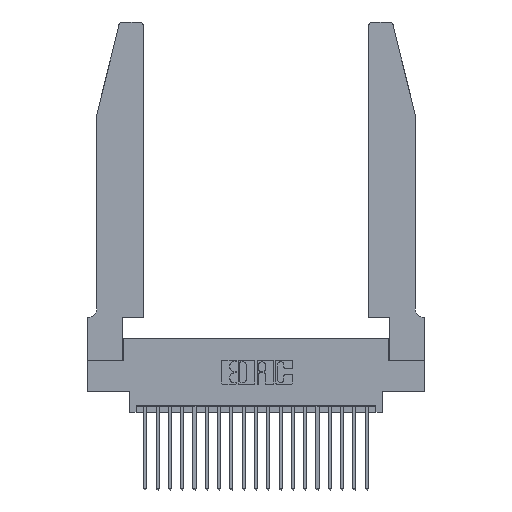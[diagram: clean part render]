
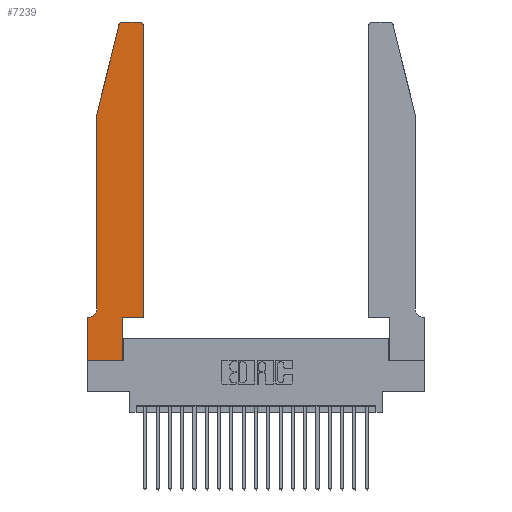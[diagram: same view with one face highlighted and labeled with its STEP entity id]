
A CAD part, top view. The second image highlights one B-rep face of the part: STEP entity #7239.
In plain terms, the highlighted planar face has unit normal (0, 0, 1).
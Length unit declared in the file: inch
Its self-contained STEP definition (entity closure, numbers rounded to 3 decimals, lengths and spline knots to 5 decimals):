
#53 = EDGE_CURVE ( 'NONE', #16785, #1456, #14814, .T. ) ;
#444 = EDGE_CURVE ( 'NONE', #21733, #634, #7860, .T. ) ;
#532 = VECTOR ( 'NONE', #2374, 39.37008 ) ;
#634 = VERTEX_POINT ( 'NONE', #20875 ) ;
#660 = ORIENTED_EDGE ( 'NONE', *, *, #5342, .T. ) ;
#842 = ORIENTED_EDGE ( 'NONE', *, *, #3606, .T. ) ;
#1038 = DIRECTION ( 'NONE',  ( 1., 0., 0. ) ) ;
#1308 = LINE ( 'NONE', #10393, #10148 ) ;
#1456 = VERTEX_POINT ( 'NONE', #11533 ) ;
#1581 = VERTEX_POINT ( 'NONE', #22406 ) ;
#1708 = AXIS2_PLACEMENT_3D ( 'NONE', #15107, #22049, #1038 ) ;
#1894 = LINE ( 'NONE', #17674, #11570 ) ;
#2374 = DIRECTION ( 'NONE',  ( 0., -1., 0. ) ) ;
#2463 = ORIENTED_EDGE ( 'NONE', *, *, #5434, .T. ) ;
#2608 = VECTOR ( 'NONE', #3742, 39.37008 ) ;
#2721 = DIRECTION ( 'NONE',  ( 1., 0., 0. ) ) ;
#3547 = EDGE_CURVE ( 'NONE', #13281, #9578, #3882, .T. ) ;
#3550 = ORIENTED_EDGE ( 'NONE', *, *, #53, .T. ) ;
#3606 = EDGE_CURVE ( 'NONE', #634, #3725, #22374, .T. ) ;
#3725 = VERTEX_POINT ( 'NONE', #6232 ) ;
#3742 = DIRECTION ( 'NONE',  ( -1., 0., 0. ) ) ;
#3859 = VERTEX_POINT ( 'NONE', #18999 ) ;
#3866 = VECTOR ( 'NONE', #10265, 39.37008 ) ;
#3882 = CIRCLE ( 'NONE', #7506, 0.03 ) ;
#4142 = ORIENTED_EDGE ( 'NONE', *, *, #4874, .T. ) ;
#4759 = CARTESIAN_POINT ( 'NONE',  ( 0.4505, 2.72, 0.37 ) ) ;
#4874 = EDGE_CURVE ( 'NONE', #1456, #13281, #1894, .T. ) ;
#5218 = DIRECTION ( 'NONE',  ( -0.239, -0.971, 0. ) ) ;
#5234 = LINE ( 'NONE', #17167, #3866 ) ;
#5342 = EDGE_CURVE ( 'NONE', #13458, #5376, #5234, .T. ) ;
#5376 = VERTEX_POINT ( 'NONE', #13996 ) ;
#5434 = EDGE_CURVE ( 'NONE', #3725, #13458, #5494, .T. ) ;
#5494 = LINE ( 'NONE', #6932, #11308 ) ;
#5713 = CARTESIAN_POINT ( 'NONE',  ( 0.0755, 0.42, 0.37 ) ) ;
#6232 = CARTESIAN_POINT ( 'NONE',  ( 0., 0., 0.37 ) ) ;
#6354 = EDGE_CURVE ( 'NONE', #9578, #3859, #1308, .T. ) ;
#6702 = EDGE_LOOP ( 'NONE', ( #4142, #7648, #18401, #22657, #6912, #9147, #842, #2463, #660, #22860, #15437, #3550 ) ) ;
#6714 = CARTESIAN_POINT ( 'NONE',  ( 0.2865, 0., 0.37 ) ) ;
#6912 = ORIENTED_EDGE ( 'NONE', *, *, #7678, .T. ) ;
#6932 = CARTESIAN_POINT ( 'NONE',  ( 0., 0., 0.37 ) ) ;
#7239 = ADVANCED_FACE ( 'NONE', ( #18969 ), #7376, .T. ) ;
#7376 = PLANE ( 'NONE',  #9772 ) ;
#7421 = CARTESIAN_POINT ( 'NONE',  ( 0.0755, 0.35, 0.37 ) ) ;
#7506 = AXIS2_PLACEMENT_3D ( 'NONE', #21258, #10679, #17708 ) ;
#7648 = ORIENTED_EDGE ( 'NONE', *, *, #3547, .T. ) ;
#7678 = EDGE_CURVE ( 'NONE', #16403, #21733, #15916, .T. ) ;
#7860 = LINE ( 'NONE', #7421, #2608 ) ;
#7906 = EDGE_CURVE ( 'NONE', #5376, #1581, #19776, .T. ) ;
#8090 = DIRECTION ( 'NONE',  ( 0., -1., 0. ) ) ;
#8780 = AXIS2_PLACEMENT_3D ( 'NONE', #10728, #22035, #14647 ) ;
#8849 = LINE ( 'NONE', #22596, #22672 ) ;
#9045 = DIRECTION ( 'NONE',  ( 1., 0., 0. ) ) ;
#9114 = CARTESIAN_POINT ( 'NONE',  ( 0., 0., 0.37 ) ) ;
#9147 = ORIENTED_EDGE ( 'NONE', *, *, #444, .T. ) ;
#9332 = CARTESIAN_POINT ( 'NONE',  ( 0.0055, 0.35, 0.37 ) ) ;
#9578 = VERTEX_POINT ( 'NONE', #19442 ) ;
#9772 = AXIS2_PLACEMENT_3D ( 'NONE', #19693, #18348, #13043 ) ;
#10148 = VECTOR ( 'NONE', #5218, 39.37008 ) ;
#10265 = DIRECTION ( 'NONE',  ( 0., 1., 0. ) ) ;
#10393 = CARTESIAN_POINT ( 'NONE',  ( 0.0755, 2., 0.37 ) ) ;
#10626 = CARTESIAN_POINT ( 'NONE',  ( 0.284, 2.75, 0.37 ) ) ;
#10679 = DIRECTION ( 'NONE',  ( 0., 0., 1. ) ) ;
#10728 = CARTESIAN_POINT ( 'NONE',  ( 0.0055, 0.42, 0.37 ) ) ;
#11308 = VECTOR ( 'NONE', #9045, 39.37008 ) ;
#11533 = CARTESIAN_POINT ( 'NONE',  ( 0.4205, 2.75, 0.37 ) ) ;
#11570 = VECTOR ( 'NONE', #21225, 39.37008 ) ;
#12288 = EDGE_CURVE ( 'NONE', #3859, #16403, #16810, .T. ) ;
#12691 = VECTOR ( 'NONE', #8090, 39.37008 ) ;
#13043 = DIRECTION ( 'NONE',  ( 1., 0., 0. ) ) ;
#13281 = VERTEX_POINT ( 'NONE', #10626 ) ;
#13458 = VERTEX_POINT ( 'NONE', #6714 ) ;
#13996 = CARTESIAN_POINT ( 'NONE',  ( 0.2865, 0.35, 0.37 ) ) ;
#14112 = DIRECTION ( 'NONE',  ( 0., 1., 0. ) ) ;
#14304 = CARTESIAN_POINT ( 'NONE',  ( 0.4505, 0.35, 0.37 ) ) ;
#14524 = VECTOR ( 'NONE', #2721, 39.37008 ) ;
#14647 = DIRECTION ( 'NONE',  ( -1., 0., 0. ) ) ;
#14814 = CIRCLE ( 'NONE', #1708, 0.03 ) ;
#15107 = CARTESIAN_POINT ( 'NONE',  ( 0.4205, 2.72, 0.37 ) ) ;
#15437 = ORIENTED_EDGE ( 'NONE', *, *, #17799, .T. ) ;
#15916 = CIRCLE ( 'NONE', #8780, 0.07 ) ;
#16403 = VERTEX_POINT ( 'NONE', #5713 ) ;
#16785 = VERTEX_POINT ( 'NONE', #4759 ) ;
#16810 = LINE ( 'NONE', #18931, #12691 ) ;
#17167 = CARTESIAN_POINT ( 'NONE',  ( 0.2865, 0.35, 0.37 ) ) ;
#17674 = CARTESIAN_POINT ( 'NONE',  ( 0.2605, 2.75, 0.37 ) ) ;
#17708 = DIRECTION ( 'NONE',  ( 1., 0., 0. ) ) ;
#17799 = EDGE_CURVE ( 'NONE', #1581, #16785, #8849, .T. ) ;
#18348 = DIRECTION ( 'NONE',  ( 0., 0., 1. ) ) ;
#18401 = ORIENTED_EDGE ( 'NONE', *, *, #6354, .T. ) ;
#18931 = CARTESIAN_POINT ( 'NONE',  ( 0.0755, 2., 0.37 ) ) ;
#18969 = FACE_OUTER_BOUND ( 'NONE', #6702, .T. ) ;
#18999 = CARTESIAN_POINT ( 'NONE',  ( 0.0755, 2., 0.37 ) ) ;
#19442 = CARTESIAN_POINT ( 'NONE',  ( 0.25487, 2.72718, 0.37 ) ) ;
#19693 = CARTESIAN_POINT ( 'NONE',  ( 0., 0.35, 0.37 ) ) ;
#19776 = LINE ( 'NONE', #14304, #14524 ) ;
#20875 = CARTESIAN_POINT ( 'NONE',  ( 0., 0.35, 0.37 ) ) ;
#21225 = DIRECTION ( 'NONE',  ( -1., 0., 0. ) ) ;
#21258 = CARTESIAN_POINT ( 'NONE',  ( 0.284, 2.72, 0.37 ) ) ;
#21733 = VERTEX_POINT ( 'NONE', #9332 ) ;
#22035 = DIRECTION ( 'NONE',  ( 0., 0., -1. ) ) ;
#22049 = DIRECTION ( 'NONE',  ( 0., 0., 1. ) ) ;
#22374 = LINE ( 'NONE', #9114, #532 ) ;
#22406 = CARTESIAN_POINT ( 'NONE',  ( 0.4505, 0.35, 0.37 ) ) ;
#22596 = CARTESIAN_POINT ( 'NONE',  ( 0.4505, 0.35, 0.37 ) ) ;
#22657 = ORIENTED_EDGE ( 'NONE', *, *, #12288, .T. ) ;
#22672 = VECTOR ( 'NONE', #14112, 39.37008 ) ;
#22860 = ORIENTED_EDGE ( 'NONE', *, *, #7906, .T. ) ;
